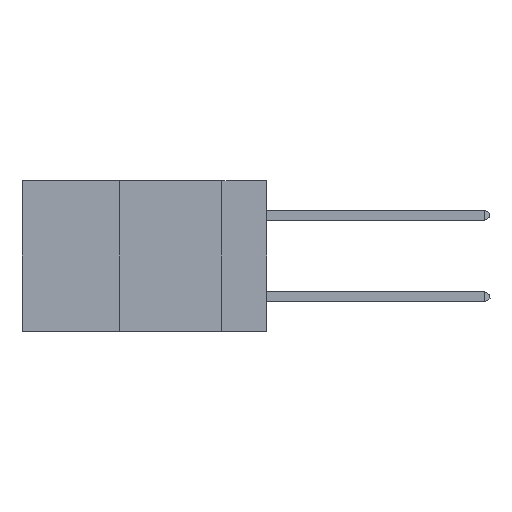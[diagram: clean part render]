
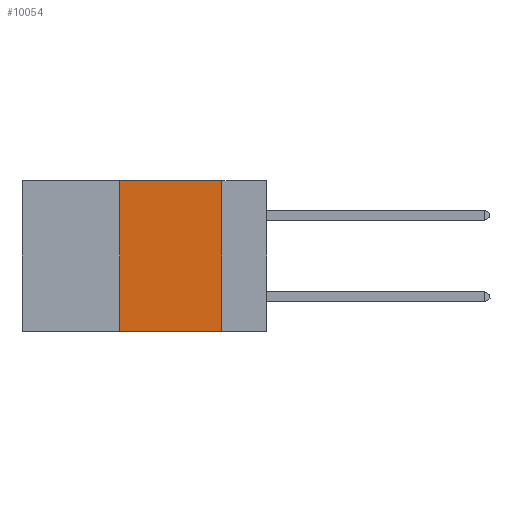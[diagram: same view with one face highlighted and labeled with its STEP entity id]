
A CAD part, left-side view. The second image highlights one B-rep face of the part: STEP entity #10054.
In plain terms, the highlighted planar face has unit normal (-1, 0, 0).
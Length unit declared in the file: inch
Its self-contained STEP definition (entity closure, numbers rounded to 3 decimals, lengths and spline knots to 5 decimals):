
#83 = CARTESIAN_POINT ( 'NONE',  ( 0., 0.6, 0. ) ) ;
#353 = LINE ( 'NONE', #3497, #3861 ) ;
#1003 = FACE_OUTER_BOUND ( 'NONE', #8784, .T. ) ;
#1216 = ORIENTED_EDGE ( 'NONE', *, *, #13904, .F. ) ;
#1383 = VECTOR ( 'NONE', #2766, 39.37008 ) ;
#1589 = DIRECTION ( 'NONE',  ( 0., -1., 0. ) ) ;
#1928 = CARTESIAN_POINT ( 'NONE',  ( 0., 0.36, 0. ) ) ;
#1936 = VERTEX_POINT ( 'NONE', #16626 ) ;
#2766 = DIRECTION ( 'NONE',  ( 0., 0., -1. ) ) ;
#3375 = CARTESIAN_POINT ( 'NONE',  ( 0., 0.11, -0.37 ) ) ;
#3497 = CARTESIAN_POINT ( 'NONE',  ( 0., 0.6, -0.37 ) ) ;
#3779 = VECTOR ( 'NONE', #1589, 39.37008 ) ;
#3861 = VECTOR ( 'NONE', #18564, 39.37008 ) ;
#4265 = VERTEX_POINT ( 'NONE', #3375 ) ;
#4952 = DIRECTION ( 'NONE',  ( 0., 0., 1. ) ) ;
#5073 = AXIS2_PLACEMENT_3D ( 'NONE', #13663, #18099, #9133 ) ;
#6828 = ORIENTED_EDGE ( 'NONE', *, *, #12291, .F. ) ;
#7270 = VERTEX_POINT ( 'NONE', #9287 ) ;
#7275 = CARTESIAN_POINT ( 'NONE',  ( 0., 0.11, 0. ) ) ;
#7869 = LINE ( 'NONE', #1928, #19412 ) ;
#8784 = EDGE_LOOP ( 'NONE', ( #6828, #12108, #1216, #16088 ) ) ;
#9133 = DIRECTION ( 'NONE',  ( 0., 0., -1. ) ) ;
#9287 = CARTESIAN_POINT ( 'NONE',  ( 0., 0.36, 0. ) ) ;
#9890 = LINE ( 'NONE', #7275, #1383 ) ;
#10054 = ADVANCED_FACE ( 'NONE', ( #1003 ), #15115, .F. ) ;
#10743 = EDGE_CURVE ( 'NONE', #7270, #1936, #16284, .T. ) ;
#12108 = ORIENTED_EDGE ( 'NONE', *, *, #10743, .F. ) ;
#12291 = EDGE_CURVE ( 'NONE', #1936, #4265, #9890, .T. ) ;
#13101 = VERTEX_POINT ( 'NONE', #15202 ) ;
#13663 = CARTESIAN_POINT ( 'NONE',  ( 0., 0.6, 0. ) ) ;
#13904 = EDGE_CURVE ( 'NONE', #13101, #7270, #7869, .T. ) ;
#13935 = EDGE_CURVE ( 'NONE', #13101, #4265, #353, .T. ) ;
#15115 = PLANE ( 'NONE',  #5073 ) ;
#15202 = CARTESIAN_POINT ( 'NONE',  ( 0., 0.36, -0.37 ) ) ;
#16088 = ORIENTED_EDGE ( 'NONE', *, *, #13935, .T. ) ;
#16284 = LINE ( 'NONE', #83, #3779 ) ;
#16626 = CARTESIAN_POINT ( 'NONE',  ( 0., 0.11, 0. ) ) ;
#18099 = DIRECTION ( 'NONE',  ( 1., 0., 0. ) ) ;
#18564 = DIRECTION ( 'NONE',  ( 0., -1., 0. ) ) ;
#19412 = VECTOR ( 'NONE', #4952, 39.37008 ) ;
